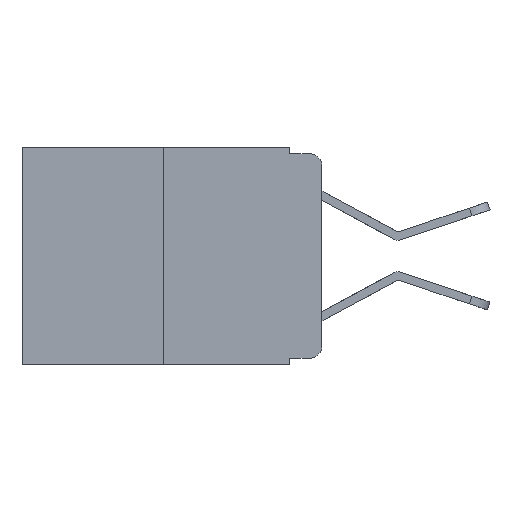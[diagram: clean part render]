
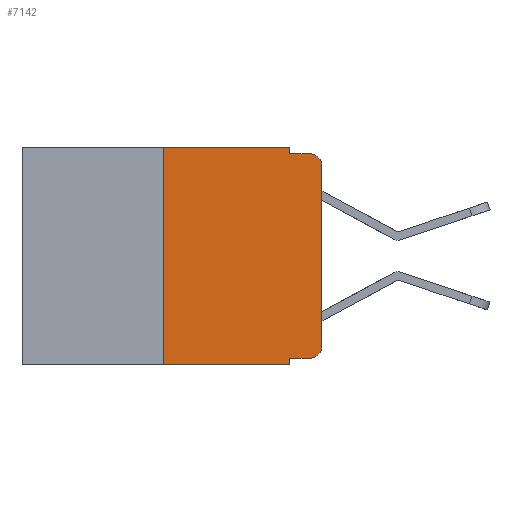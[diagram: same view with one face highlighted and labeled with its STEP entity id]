
A CAD part, left-side view. The second image highlights one B-rep face of the part: STEP entity #7142.
In plain terms, the highlighted planar face has unit normal (-1, 0, 0).
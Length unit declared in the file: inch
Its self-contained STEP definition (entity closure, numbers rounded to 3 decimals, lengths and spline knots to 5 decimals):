
#1 = DIRECTION ( 'NONE',  ( 0., 0., -1. ) ) ;
#109 = EDGE_CURVE ( 'NONE', #5588, #9831, #10017, .T. ) ;
#448 = VERTEX_POINT ( 'NONE', #1668 ) ;
#650 = LINE ( 'NONE', #8809, #4917 ) ;
#673 = DIRECTION ( 'NONE',  ( 0., 0., -1. ) ) ;
#748 = EDGE_CURVE ( 'NONE', #6097, #2385, #8946, .T. ) ;
#837 = VECTOR ( 'NONE', #6832, 39.37008 ) ;
#838 = DIRECTION ( 'NONE',  ( 0., 0., 1. ) ) ;
#1157 = EDGE_LOOP ( 'NONE', ( #7241, #1743, #5095, #9044, #5892, #1998, #4244, #7327, #5221, #3670 ) ) ;
#1369 = VECTOR ( 'NONE', #673, 39.37008 ) ;
#1416 = DIRECTION ( 'NONE',  ( 1., 0., 0. ) ) ;
#1522 = CARTESIAN_POINT ( 'NONE',  ( 0., 0.473, 0. ) ) ;
#1626 = LINE ( 'NONE', #4236, #8486 ) ;
#1668 = CARTESIAN_POINT ( 'NONE',  ( 0., 0.051, 0. ) ) ;
#1743 = ORIENTED_EDGE ( 'NONE', *, *, #748, .T. ) ;
#1802 = CARTESIAN_POINT ( 'NONE',  ( 0., 0.25, 0. ) ) ;
#1968 = EDGE_CURVE ( 'NONE', #2658, #6097, #5791, .T. ) ;
#1998 = ORIENTED_EDGE ( 'NONE', *, *, #4107, .F. ) ;
#2111 = VECTOR ( 'NONE', #10054, 39.37008 ) ;
#2148 = CARTESIAN_POINT ( 'NONE',  ( 0., 0.02, -0.03 ) ) ;
#2170 = DIRECTION ( 'NONE',  ( 0., 0., -1. ) ) ;
#2186 = CARTESIAN_POINT ( 'NONE',  ( 0., 0., -0.313 ) ) ;
#2285 = DIRECTION ( 'NONE',  ( -1., 0., 0. ) ) ;
#2324 = DIRECTION ( 'NONE',  ( 0., 0., -1. ) ) ;
#2335 = AXIS2_PLACEMENT_3D ( 'NONE', #2148, #2285, #2324 ) ;
#2385 = VERTEX_POINT ( 'NONE', #9555 ) ;
#2658 = VERTEX_POINT ( 'NONE', #2186 ) ;
#2817 = CARTESIAN_POINT ( 'NONE',  ( 0., 0.02, -0.313 ) ) ;
#2976 = EDGE_CURVE ( 'NONE', #9831, #2658, #4670, .T. ) ;
#3384 = DIRECTION ( 'NONE',  ( 0., -1., 0. ) ) ;
#3477 = PLANE ( 'NONE',  #7772 ) ;
#3664 = CARTESIAN_POINT ( 'NONE',  ( 0., 0.25, 0. ) ) ;
#3670 = ORIENTED_EDGE ( 'NONE', *, *, #2976, .T. ) ;
#3701 = DIRECTION ( 'NONE',  ( 0., 0., -1. ) ) ;
#3803 = EDGE_CURVE ( 'NONE', #4351, #5005, #650, .T. ) ;
#4107 = EDGE_CURVE ( 'NONE', #4351, #7495, #4210, .T. ) ;
#4143 = CARTESIAN_POINT ( 'NONE',  ( 0., 0.051, -0.01 ) ) ;
#4210 = LINE ( 'NONE', #3664, #2111 ) ;
#4236 = CARTESIAN_POINT ( 'NONE',  ( 0., 0.473, 0. ) ) ;
#4244 = ORIENTED_EDGE ( 'NONE', *, *, #3803, .T. ) ;
#4266 = CARTESIAN_POINT ( 'NONE',  ( 0., 0.051, -0.343 ) ) ;
#4334 = EDGE_CURVE ( 'NONE', #448, #7208, #8263, .T. ) ;
#4351 = VERTEX_POINT ( 'NONE', #10490 ) ;
#4660 = CARTESIAN_POINT ( 'NONE',  ( 0., 0.051, 0. ) ) ;
#4670 = CIRCLE ( 'NONE', #6755, 0.02 ) ;
#4917 = VECTOR ( 'NONE', #6670, 39.37008 ) ;
#5005 = VERTEX_POINT ( 'NONE', #4266 ) ;
#5095 = ORIENTED_EDGE ( 'NONE', *, *, #9206, .F. ) ;
#5106 = CARTESIAN_POINT ( 'NONE',  ( 0., 0., 0. ) ) ;
#5119 = LINE ( 'NONE', #11209, #7225 ) ;
#5221 = ORIENTED_EDGE ( 'NONE', *, *, #109, .T. ) ;
#5588 = VERTEX_POINT ( 'NONE', #7363 ) ;
#5791 = LINE ( 'NONE', #5106, #9905 ) ;
#5892 = ORIENTED_EDGE ( 'NONE', *, *, #6786, .F. ) ;
#5993 = CARTESIAN_POINT ( 'NONE',  ( 0., 0.02, -0.333 ) ) ;
#6097 = VERTEX_POINT ( 'NONE', #9152 ) ;
#6659 = CARTESIAN_POINT ( 'NONE',  ( 0., 0.051, -0.333 ) ) ;
#6670 = DIRECTION ( 'NONE',  ( 0., -1., 0. ) ) ;
#6755 = AXIS2_PLACEMENT_3D ( 'NONE', #2817, #9026, #3701 ) ;
#6786 = EDGE_CURVE ( 'NONE', #7495, #448, #1626, .T. ) ;
#6832 = DIRECTION ( 'NONE',  ( 0., -1., 0. ) ) ;
#7126 = CARTESIAN_POINT ( 'NONE',  ( 0., 0.051, 0. ) ) ;
#7142 = ADVANCED_FACE ( 'NONE', ( #10190 ), #3477, .F. ) ;
#7208 = VERTEX_POINT ( 'NONE', #4143 ) ;
#7225 = VECTOR ( 'NONE', #3384, 39.37008 ) ;
#7241 = ORIENTED_EDGE ( 'NONE', *, *, #1968, .T. ) ;
#7327 = ORIENTED_EDGE ( 'NONE', *, *, #8869, .F. ) ;
#7363 = CARTESIAN_POINT ( 'NONE',  ( 0., 0.051, -0.333 ) ) ;
#7495 = VERTEX_POINT ( 'NONE', #1802 ) ;
#7772 = AXIS2_PLACEMENT_3D ( 'NONE', #1522, #1416, #2170 ) ;
#8215 = LINE ( 'NONE', #7126, #10449 ) ;
#8263 = LINE ( 'NONE', #4660, #1369 ) ;
#8486 = VECTOR ( 'NONE', #10894, 39.37008 ) ;
#8809 = CARTESIAN_POINT ( 'NONE',  ( 0., 0.473, -0.343 ) ) ;
#8869 = EDGE_CURVE ( 'NONE', #5588, #5005, #8215, .T. ) ;
#8946 = CIRCLE ( 'NONE', #2335, 0.02 ) ;
#9026 = DIRECTION ( 'NONE',  ( -1., 0., 0. ) ) ;
#9044 = ORIENTED_EDGE ( 'NONE', *, *, #4334, .F. ) ;
#9152 = CARTESIAN_POINT ( 'NONE',  ( 0., 0., -0.03 ) ) ;
#9206 = EDGE_CURVE ( 'NONE', #7208, #2385, #5119, .T. ) ;
#9555 = CARTESIAN_POINT ( 'NONE',  ( 0., 0.02, -0.01 ) ) ;
#9831 = VERTEX_POINT ( 'NONE', #5993 ) ;
#9905 = VECTOR ( 'NONE', #838, 39.37008 ) ;
#10017 = LINE ( 'NONE', #6659, #837 ) ;
#10054 = DIRECTION ( 'NONE',  ( 0., 0., 1. ) ) ;
#10190 = FACE_OUTER_BOUND ( 'NONE', #1157, .T. ) ;
#10449 = VECTOR ( 'NONE', #1, 39.37008 ) ;
#10490 = CARTESIAN_POINT ( 'NONE',  ( 0., 0.25, -0.343 ) ) ;
#10894 = DIRECTION ( 'NONE',  ( 0., -1., 0. ) ) ;
#11209 = CARTESIAN_POINT ( 'NONE',  ( 0., 0.051, -0.01 ) ) ;
